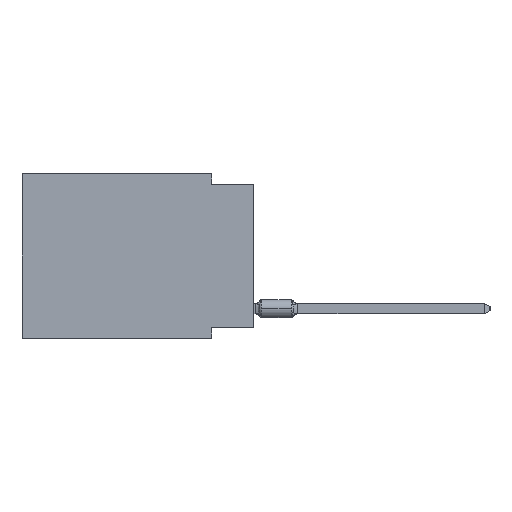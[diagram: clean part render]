
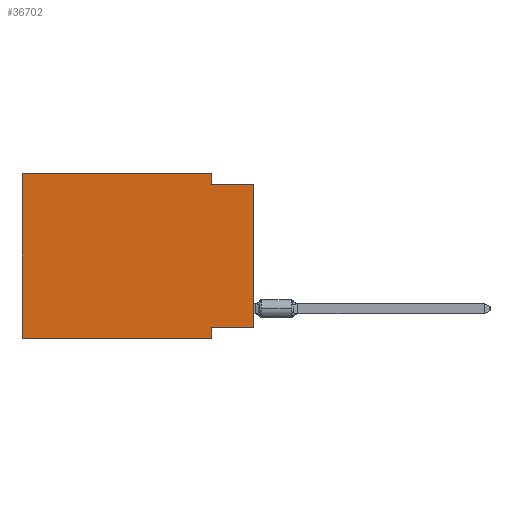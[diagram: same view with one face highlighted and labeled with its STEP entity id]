
A CAD part, left-side view. The second image highlights one B-rep face of the part: STEP entity #36702.
In plain terms, the highlighted planar face has unit normal (-1, 0, 0).
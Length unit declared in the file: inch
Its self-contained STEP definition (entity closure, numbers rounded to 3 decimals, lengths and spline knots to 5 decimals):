
#239 = CARTESIAN_POINT ( 'NONE',  ( 0., 0., -0.365 ) ) ;
#880 = DIRECTION ( 'NONE',  ( 0., 0., -1. ) ) ;
#1177 = CARTESIAN_POINT ( 'NONE',  ( 0., 0.1, -0.39 ) ) ;
#1563 = VERTEX_POINT ( 'NONE', #39483 ) ;
#1996 = LINE ( 'NONE', #70489, #19542 ) ;
#2303 = DIRECTION ( 'NONE',  ( 0., 0., -1. ) ) ;
#2481 = EDGE_CURVE ( 'NONE', #50738, #30960, #30532, .T. ) ;
#2593 = ORIENTED_EDGE ( 'NONE', *, *, #19315, .T. ) ;
#2688 = LINE ( 'NONE', #36542, #39503 ) ;
#3614 = ORIENTED_EDGE ( 'NONE', *, *, #62398, .F. ) ;
#4610 = CARTESIAN_POINT ( 'NONE',  ( 0., 0., -0.365 ) ) ;
#5732 = VECTOR ( 'NONE', #10545, 39.37008 ) ;
#8231 = DIRECTION ( 'NONE',  ( 0., 0., 1. ) ) ;
#10039 = VERTEX_POINT ( 'NONE', #11935 ) ;
#10545 = DIRECTION ( 'NONE',  ( 0., -1., 0. ) ) ;
#11527 = VECTOR ( 'NONE', #8231, 39.37008 ) ;
#11578 = ORIENTED_EDGE ( 'NONE', *, *, #29852, .F. ) ;
#11935 = CARTESIAN_POINT ( 'NONE',  ( 0., 0.1, 0. ) ) ;
#15493 = CARTESIAN_POINT ( 'NONE',  ( 0., 0.55, 0. ) ) ;
#16192 = LINE ( 'NONE', #62095, #5732 ) ;
#16430 = VERTEX_POINT ( 'NONE', #27450 ) ;
#19315 = EDGE_CURVE ( 'NONE', #52500, #16430, #2688, .T. ) ;
#19542 = VECTOR ( 'NONE', #880, 39.37008 ) ;
#21354 = EDGE_CURVE ( 'NONE', #1563, #30960, #34195, .T. ) ;
#23263 = PLANE ( 'NONE',  #57560 ) ;
#23862 = CARTESIAN_POINT ( 'NONE',  ( 0., 0.1, -0.025 ) ) ;
#25633 = DIRECTION ( 'NONE',  ( 0., 0., 1. ) ) ;
#26180 = CARTESIAN_POINT ( 'NONE',  ( 0., 0.1, -0.39 ) ) ;
#26298 = CARTESIAN_POINT ( 'NONE',  ( 0., 0.1, -0.365 ) ) ;
#27450 = CARTESIAN_POINT ( 'NONE',  ( 0., 0., -0.025 ) ) ;
#28106 = ORIENTED_EDGE ( 'NONE', *, *, #31610, .F. ) ;
#29619 = VERTEX_POINT ( 'NONE', #23862 ) ;
#29852 = EDGE_CURVE ( 'NONE', #52500, #50738, #56180, .T. ) ;
#30532 = LINE ( 'NONE', #1177, #37212 ) ;
#30960 = VERTEX_POINT ( 'NONE', #26180 ) ;
#31345 = VECTOR ( 'NONE', #52251, 39.37008 ) ;
#31610 = EDGE_CURVE ( 'NONE', #1563, #49715, #71848, .T. ) ;
#31780 = VECTOR ( 'NONE', #50520, 39.37008 ) ;
#32967 = ORIENTED_EDGE ( 'NONE', *, *, #43617, .F. ) ;
#34195 = LINE ( 'NONE', #58649, #31345 ) ;
#36542 = CARTESIAN_POINT ( 'NONE',  ( 0., 0., 0. ) ) ;
#36702 = ADVANCED_FACE ( 'NONE', ( #39456 ), #23263, .F. ) ;
#37212 = VECTOR ( 'NONE', #2303, 39.37008 ) ;
#37648 = ORIENTED_EDGE ( 'NONE', *, *, #21354, .T. ) ;
#39456 = FACE_OUTER_BOUND ( 'NONE', #48268, .T. ) ;
#39483 = CARTESIAN_POINT ( 'NONE',  ( 0., 0.55, -0.39 ) ) ;
#39503 = VECTOR ( 'NONE', #25633, 39.37008 ) ;
#43617 = EDGE_CURVE ( 'NONE', #49715, #10039, #16192, .T. ) ;
#44157 = ORIENTED_EDGE ( 'NONE', *, *, #71216, .F. ) ;
#46214 = DIRECTION ( 'NONE',  ( 1., 0., 0. ) ) ;
#48268 = EDGE_LOOP ( 'NONE', ( #2593, #3614, #44157, #32967, #28106, #37648, #57396, #11578 ) ) ;
#48561 = LINE ( 'NONE', #70148, #69758 ) ;
#49715 = VERTEX_POINT ( 'NONE', #15493 ) ;
#50520 = DIRECTION ( 'NONE',  ( 0., 1., 0. ) ) ;
#50738 = VERTEX_POINT ( 'NONE', #26298 ) ;
#52251 = DIRECTION ( 'NONE',  ( 0., -1., 0. ) ) ;
#52500 = VERTEX_POINT ( 'NONE', #239 ) ;
#54226 = DIRECTION ( 'NONE',  ( 0., -1., 0. ) ) ;
#56180 = LINE ( 'NONE', #4610, #31780 ) ;
#57396 = ORIENTED_EDGE ( 'NONE', *, *, #2481, .F. ) ;
#57560 = AXIS2_PLACEMENT_3D ( 'NONE', #62779, #46214, #69171 ) ;
#58649 = CARTESIAN_POINT ( 'NONE',  ( 0., 0.55, -0.39 ) ) ;
#59801 = CARTESIAN_POINT ( 'NONE',  ( 0., 0.55, 0. ) ) ;
#62095 = CARTESIAN_POINT ( 'NONE',  ( 0., 0.55, 0. ) ) ;
#62398 = EDGE_CURVE ( 'NONE', #29619, #16430, #48561, .T. ) ;
#62779 = CARTESIAN_POINT ( 'NONE',  ( 0., 0.55, 0. ) ) ;
#69171 = DIRECTION ( 'NONE',  ( 0., 0., -1. ) ) ;
#69758 = VECTOR ( 'NONE', #54226, 39.37008 ) ;
#70148 = CARTESIAN_POINT ( 'NONE',  ( 0., 0., -0.025 ) ) ;
#70489 = CARTESIAN_POINT ( 'NONE',  ( 0., 0.1, 0. ) ) ;
#71216 = EDGE_CURVE ( 'NONE', #10039, #29619, #1996, .T. ) ;
#71848 = LINE ( 'NONE', #59801, #11527 ) ;
